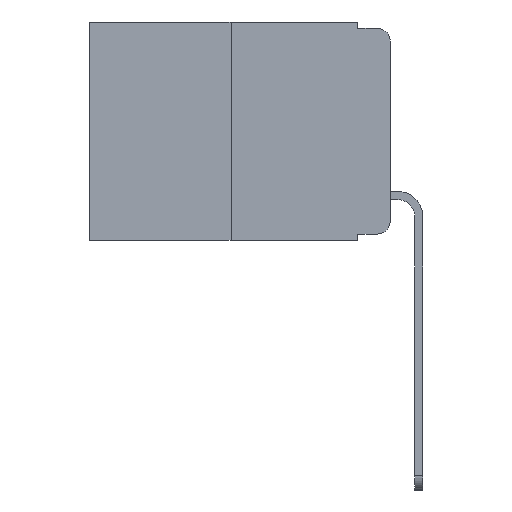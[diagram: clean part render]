
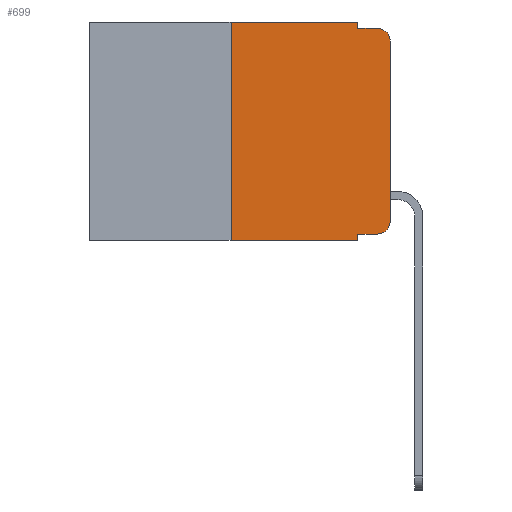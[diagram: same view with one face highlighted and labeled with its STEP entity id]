
A CAD part, left-side view. The second image highlights one B-rep face of the part: STEP entity #699.
In plain terms, the highlighted planar face has unit normal (-1, 0, 0).
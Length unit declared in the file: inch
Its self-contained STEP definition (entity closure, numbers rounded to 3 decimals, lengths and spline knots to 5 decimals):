
#121 = ORIENTED_EDGE ( 'NONE', *, *, #432, .F. ) ;
#367 = PLANE ( 'NONE',  #16256 ) ;
#427 = VERTEX_POINT ( 'NONE', #13747 ) ;
#432 = EDGE_CURVE ( 'NONE', #13838, #427, #17369, .T. ) ;
#666 = FACE_OUTER_BOUND ( 'NONE', #1048, .T. ) ;
#699 = ADVANCED_FACE ( 'NONE', ( #666 ), #367, .F. ) ;
#977 = VERTEX_POINT ( 'NONE', #12648 ) ;
#1048 = EDGE_LOOP ( 'NONE', ( #4453, #3871, #17460, #17391, #7080, #8127, #5061, #121, #7890, #13901 ) ) ;
#2444 = EDGE_CURVE ( 'NONE', #25022, #4445, #18755, .T. ) ;
#2625 = EDGE_CURVE ( 'NONE', #14281, #427, #9634, .T. ) ;
#3048 = CARTESIAN_POINT ( 'NONE',  ( 0., 0.02, -0.313 ) ) ;
#3871 = ORIENTED_EDGE ( 'NONE', *, *, #8153, .T. ) ;
#4445 = VERTEX_POINT ( 'NONE', #8394 ) ;
#4453 = ORIENTED_EDGE ( 'NONE', *, *, #16153, .T. ) ;
#4518 = VECTOR ( 'NONE', #19958, 39.37008 ) ;
#4788 = CARTESIAN_POINT ( 'NONE',  ( 0., 0.051, 0. ) ) ;
#5061 = ORIENTED_EDGE ( 'NONE', *, *, #2625, .T. ) ;
#5096 = CARTESIAN_POINT ( 'NONE',  ( 0., 0.25, -0.343 ) ) ;
#5103 = LINE ( 'NONE', #13826, #9306 ) ;
#5449 = CARTESIAN_POINT ( 'NONE',  ( 0., 0.051, -0.333 ) ) ;
#5463 = VERTEX_POINT ( 'NONE', #6061 ) ;
#5998 = CARTESIAN_POINT ( 'NONE',  ( 0., 0.051, -0.01 ) ) ;
#6061 = CARTESIAN_POINT ( 'NONE',  ( 0., 0., -0.313 ) ) ;
#6405 = CARTESIAN_POINT ( 'NONE',  ( 0., 0.02, -0.03 ) ) ;
#6761 = DIRECTION ( 'NONE',  ( 0., 0., -1. ) ) ;
#7080 = ORIENTED_EDGE ( 'NONE', *, *, #18469, .F. ) ;
#7823 = DIRECTION ( 'NONE',  ( 0., -1., 0. ) ) ;
#7890 = ORIENTED_EDGE ( 'NONE', *, *, #19274, .T. ) ;
#8017 = DIRECTION ( 'NONE',  ( 0., 0., 1. ) ) ;
#8033 = EDGE_CURVE ( 'NONE', #14281, #24152, #24769, .T. ) ;
#8127 = ORIENTED_EDGE ( 'NONE', *, *, #8033, .F. ) ;
#8153 = EDGE_CURVE ( 'NONE', #22793, #4445, #13823, .T. ) ;
#8394 = CARTESIAN_POINT ( 'NONE',  ( 0., 0.02, -0.01 ) ) ;
#9306 = VECTOR ( 'NONE', #7823, 39.37008 ) ;
#9634 = LINE ( 'NONE', #17927, #4518 ) ;
#10138 = CARTESIAN_POINT ( 'NONE',  ( 0., 0.051, 0. ) ) ;
#10694 = CARTESIAN_POINT ( 'NONE',  ( 0., 0.25, 0. ) ) ;
#10773 = LINE ( 'NONE', #14738, #18680 ) ;
#11364 = DIRECTION ( 'NONE',  ( 0., -1., 0. ) ) ;
#11676 = CARTESIAN_POINT ( 'NONE',  ( 0., 0.25, 0. ) ) ;
#12157 = DIRECTION ( 'NONE',  ( 0., 0., 1. ) ) ;
#12354 = CARTESIAN_POINT ( 'NONE',  ( 0., 0.02, -0.333 ) ) ;
#12442 = LINE ( 'NONE', #14022, #19707 ) ;
#12648 = CARTESIAN_POINT ( 'NONE',  ( 0., 0.051, 0. ) ) ;
#13101 = EDGE_CURVE ( 'NONE', #20626, #5463, #15630, .T. ) ;
#13348 = AXIS2_PLACEMENT_3D ( 'NONE', #3048, #16586, #20469 ) ;
#13545 = EDGE_CURVE ( 'NONE', #977, #25022, #18963, .T. ) ;
#13747 = CARTESIAN_POINT ( 'NONE',  ( 0., 0.051, -0.343 ) ) ;
#13823 = CIRCLE ( 'NONE', #22202, 0.02 ) ;
#13826 = CARTESIAN_POINT ( 'NONE',  ( 0., 0.473, 0. ) ) ;
#13838 = VERTEX_POINT ( 'NONE', #5449 ) ;
#13898 = CARTESIAN_POINT ( 'NONE',  ( 0., 0.473, 0. ) ) ;
#13901 = ORIENTED_EDGE ( 'NONE', *, *, #13101, .T. ) ;
#14022 = CARTESIAN_POINT ( 'NONE',  ( 0., 0., 0. ) ) ;
#14281 = VERTEX_POINT ( 'NONE', #5096 ) ;
#14738 = CARTESIAN_POINT ( 'NONE',  ( 0., 0.051, -0.333 ) ) ;
#15630 = CIRCLE ( 'NONE', #13348, 0.02 ) ;
#16153 = EDGE_CURVE ( 'NONE', #5463, #22793, #12442, .T. ) ;
#16256 = AXIS2_PLACEMENT_3D ( 'NONE', #13898, #23832, #19834 ) ;
#16282 = DIRECTION ( 'NONE',  ( 0., 0., -1. ) ) ;
#16586 = DIRECTION ( 'NONE',  ( -1., 0., 0. ) ) ;
#17144 = CARTESIAN_POINT ( 'NONE',  ( 0., 0.051, -0.01 ) ) ;
#17369 = LINE ( 'NONE', #10138, #24956 ) ;
#17391 = ORIENTED_EDGE ( 'NONE', *, *, #13545, .F. ) ;
#17460 = ORIENTED_EDGE ( 'NONE', *, *, #2444, .F. ) ;
#17927 = CARTESIAN_POINT ( 'NONE',  ( 0., 0.473, -0.343 ) ) ;
#17935 = DIRECTION ( 'NONE',  ( 0., 0., -1. ) ) ;
#18380 = DIRECTION ( 'NONE',  ( 0., -1., 0. ) ) ;
#18469 = EDGE_CURVE ( 'NONE', #24152, #977, #5103, .T. ) ;
#18680 = VECTOR ( 'NONE', #18380, 39.37008 ) ;
#18755 = LINE ( 'NONE', #17144, #22415 ) ;
#18963 = LINE ( 'NONE', #4788, #19859 ) ;
#19274 = EDGE_CURVE ( 'NONE', #13838, #20626, #10773, .T. ) ;
#19707 = VECTOR ( 'NONE', #12157, 39.37008 ) ;
#19834 = DIRECTION ( 'NONE',  ( 0., 0., -1. ) ) ;
#19851 = CARTESIAN_POINT ( 'NONE',  ( 0., 0., -0.03 ) ) ;
#19859 = VECTOR ( 'NONE', #16282, 39.37008 ) ;
#19958 = DIRECTION ( 'NONE',  ( 0., -1., 0. ) ) ;
#20469 = DIRECTION ( 'NONE',  ( 0., 0., -1. ) ) ;
#20626 = VERTEX_POINT ( 'NONE', #12354 ) ;
#22202 = AXIS2_PLACEMENT_3D ( 'NONE', #6405, #24050, #17935 ) ;
#22415 = VECTOR ( 'NONE', #11364, 39.37008 ) ;
#22793 = VERTEX_POINT ( 'NONE', #19851 ) ;
#23832 = DIRECTION ( 'NONE',  ( 1., 0., 0. ) ) ;
#24050 = DIRECTION ( 'NONE',  ( -1., 0., 0. ) ) ;
#24152 = VERTEX_POINT ( 'NONE', #10694 ) ;
#24155 = VECTOR ( 'NONE', #8017, 39.37008 ) ;
#24769 = LINE ( 'NONE', #11676, #24155 ) ;
#24956 = VECTOR ( 'NONE', #6761, 39.37008 ) ;
#25022 = VERTEX_POINT ( 'NONE', #5998 ) ;
